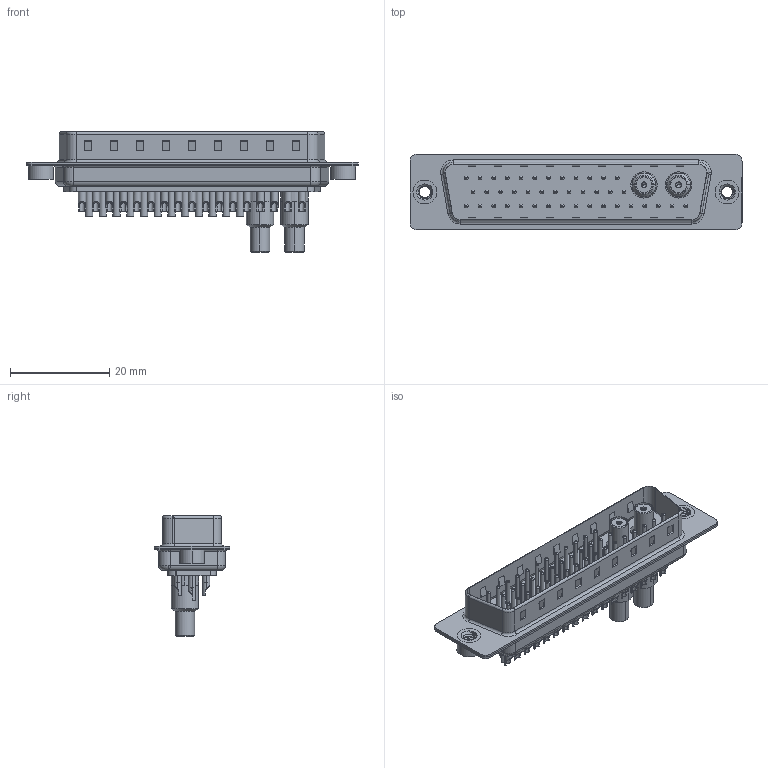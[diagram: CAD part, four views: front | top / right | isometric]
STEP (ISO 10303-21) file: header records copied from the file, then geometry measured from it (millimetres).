
FILE_DESCRIPTION (( 'STEP AP203' ), '1' );
FILE_NAME ('627-43W2222-7T2.STEP', '2019-06-19T21:54:31', ( '' ), ( '' ), 'SwSTEP 2.0', 'SolidWorks 2016', '' );
FILE_SCHEMA (( 'CONFIG_CONTROL_DESIGN' ));
Length unit declared in the file: millimetre
Products named in the file (15): 627Combo Shell Rear_50 Contacts; Co-Ax Jack Assy_SC; 627Combo Shell Front_50 Contacts; 627Combo Contact Row 1_22; 627Combo Threaded Rivet_2; 627Combo Contact Row 2_22L; Co-Ax Jack_Solder Cup Tail; 627Combo Contact Row 3_22; Insulator Socket; 627-43W2222-7T2; Insulator Socket 2; Locking Collar; Socket_Solder Cup; 627Combo Housing_43W2; Solder Cover
Assembly tree (54 placements, depth 3):
  627-43W2222-7T2
    627Combo Housing_43W2
    627Combo Shell Rear_50 Contacts
    627Combo Shell Front_50 Contacts
    627Combo Threaded Rivet_2  x2
    Co-Ax Jack Assy_SC  x2
      Co-Ax Jack_Solder Cup Tail
      Insulator Socket
      Insulator Socket 2
      Locking Collar
      Socket_Solder Cup
      Solder Cover
    627Combo Contact Row 1_22  x12
    627Combo Contact Row 2_22L  x12
    627Combo Contact Row 3_22  x17
Bounding box: 67 x 15.3 x 24.3 mm (x, y, z)
Volume: 4865.4 mm3; surface area: 12790.8 mm2
Topology: 58 solids, 58 shells, 2189 faces, 5079 edges, 3109 vertices
Faces by surface type: cylinder 925, plane 652, torus 468, cone 134, bspline 10
Entity records: 31705 total; most frequent: CARTESIAN_POINT 6363, DIRECTION 5123, ORIENTED_EDGE 4402, EDGE_CURVE 2201, AXIS2_PLACEMENT_3D 2031, VERTEX_POINT 1407, EDGE_LOOP 1184, VECTOR 1061
